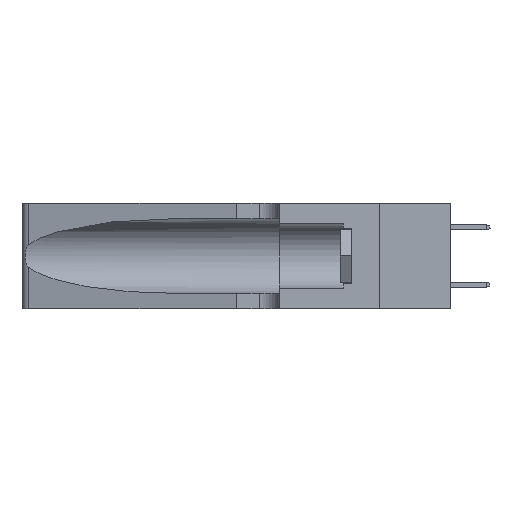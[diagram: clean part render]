
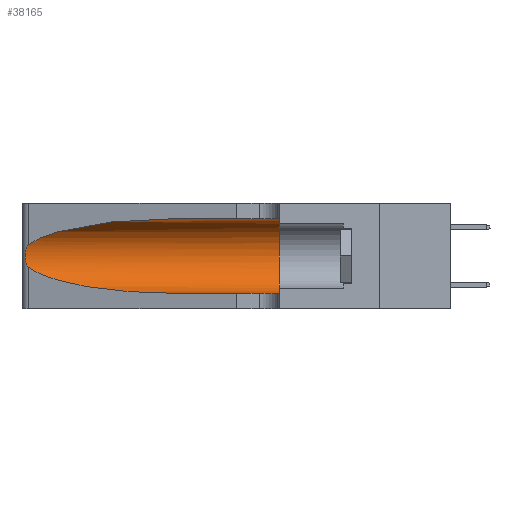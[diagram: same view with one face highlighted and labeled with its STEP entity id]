
A CAD part, left-side view. The second image highlights one B-rep face of the part: STEP entity #38165.
In plain terms, the highlighted cylindrical face has radius 3.308 mm (diameter 6.617 mm), a partial arc.
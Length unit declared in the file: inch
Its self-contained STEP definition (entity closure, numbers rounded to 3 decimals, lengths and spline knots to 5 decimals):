
#674 = CARTESIAN_POINT ( 'NONE',  ( 0.25487, 1.22718, 0.22369 ) ) ;
#1548 = CARTESIAN_POINT ( 'NONE',  ( 0.1305, 0.35, 0.31525 ) ) ;
#2005 = CARTESIAN_POINT ( 'NONE',  ( 0.1305, 1.61858, 0.05475 ) ) ;
#2157 = CARTESIAN_POINT ( 'NONE',  ( 0.2373, 1.15595, 0.08982 ) ) ;
#2640 = CARTESIAN_POINT ( 'NONE',  ( 0.18966, 0.96281, 0.31525 ) ) ;
#2766 = ORIENTED_EDGE ( 'NONE', *, *, #16112, .T. ) ;
#3418 = ORIENTED_EDGE ( 'NONE', *, *, #40777, .T. ) ;
#3511 = CARTESIAN_POINT ( 'NONE',  ( 0.26017, 1.23833, 0.17102 ) ) ;
#4199 = VERTEX_POINT ( 'NONE', #1548 ) ;
#4525 = AXIS2_PLACEMENT_3D ( 'NONE', #36823, #33344, #7733 ) ;
#6346 = CARTESIAN_POINT ( 'NONE',  ( 0.2373, 1.15595, 0.28018 ) ) ;
#6961 = CARTESIAN_POINT ( 'NONE',  ( 0.26018, 1.23835, 0.19895 ) ) ;
#7003 = VERTEX_POINT ( 'NONE', #29132 ) ;
#7064 = VERTEX_POINT ( 'NONE', #30273 ) ;
#7733 = DIRECTION ( 'NONE',  ( 0., 0., 1. ) ) ;
#8592 = EDGE_CURVE ( 'NONE', #4199, #7003, #25182, .T. ) ;
#10224 = CARTESIAN_POINT ( 'NONE',  ( 0.25789, 1.23486, 0.15765 ) ) ;
#10460 = CARTESIAN_POINT ( 'NONE',  ( 0.25555, 1.22994, 0.2215 ) ) ;
#12903 = DIRECTION ( 'NONE',  ( 0., -1., 0. ) ) ;
#13152 = DIRECTION ( 'NONE',  ( 0., 0., -1. ) ) ;
#15577 =( BOUNDED_CURVE ( )  B_SPLINE_CURVE ( 3, ( #26675, #2157, #44427, #23227 ),
 .UNSPECIFIED., .F., .F. ) 
 B_SPLINE_CURVE_WITH_KNOTS ( ( 4, 4 ),
 ( 3.44316, 4.71239 ),
 .UNSPECIFIED. ) 
 CURVE ( )  GEOMETRIC_REPRESENTATION_ITEM ( )  RATIONAL_B_SPLINE_CURVE ( ( 1., 0.87, 0.87, 1. ) ) 
 REPRESENTATION_ITEM ( '' )  );
#15943 = CARTESIAN_POINT ( 'NONE',  ( 0.1305, 1.61858, 0.185 ) ) ;
#16112 = EDGE_CURVE ( 'NONE', #7064, #22006, #23537, .T. ) ;
#16828 = VECTOR ( 'NONE', #44669, 39.37008 ) ;
#17177 = CARTESIAN_POINT ( 'NONE',  ( 0.25787, 1.23484, 0.2124 ) ) ;
#19593 = CARTESIAN_POINT ( 'NONE',  ( 0.25487, 1.22718, 0.14631 ) ) ;
#20076 = B_SPLINE_CURVE_WITH_KNOTS ( 'NONE', 3,
 ( #23890, #10460, #20635, #17177, #45322, #6961, #20409, #27554, #3511, #31676, #10224, #24324, #21318, #38618 ),
 .UNSPECIFIED., .F., .F.,
 ( 4, 2, 2, 2, 2, 2, 4 ),
 ( 0., 0.00027, 0.00053, 0.00107, 0.0016, 0.00187, 0.00214 ),
 .UNSPECIFIED. ) ;
#20228 = CARTESIAN_POINT ( 'NONE',  ( 0.25487, 1.22718, 0.22369 ) ) ;
#20409 = CARTESIAN_POINT ( 'NONE',  ( 0.26075, 1.23896, 0.19203 ) ) ;
#20635 = CARTESIAN_POINT ( 'NONE',  ( 0.25639, 1.23184, 0.21858 ) ) ;
#21318 = CARTESIAN_POINT ( 'NONE',  ( 0.25555, 1.22993, 0.14849 ) ) ;
#22006 = VERTEX_POINT ( 'NONE', #674 ) ;
#23227 = CARTESIAN_POINT ( 'NONE',  ( 0.1305, 0.72297, 0.05475 ) ) ;
#23537 =( BOUNDED_CURVE ( )  B_SPLINE_CURVE ( 3, ( #27380, #2640, #6346, #20228 ),
 .UNSPECIFIED., .F., .F. ) 
 B_SPLINE_CURVE_WITH_KNOTS ( ( 4, 4 ),
 ( 1.5708, 2.84003 ),
 .UNSPECIFIED. ) 
 CURVE ( )  GEOMETRIC_REPRESENTATION_ITEM ( )  RATIONAL_B_SPLINE_CURVE ( ( 1., 0.87, 0.87, 1. ) ) 
 REPRESENTATION_ITEM ( '' )  );
#23542 = DIRECTION ( 'NONE',  ( 0., -1., 0. ) ) ;
#23890 = CARTESIAN_POINT ( 'NONE',  ( 0.25487, 1.22718, 0.22369 ) ) ;
#24324 = CARTESIAN_POINT ( 'NONE',  ( 0.25639, 1.23186, 0.15144 ) ) ;
#24605 = EDGE_LOOP ( 'NONE', ( #2766, #3418, #42504, #27431, #30433, #39760 ) ) ;
#24941 = VERTEX_POINT ( 'NONE', #27247 ) ;
#25182 = CIRCLE ( 'NONE', #4525, 0.13025 ) ;
#26675 = CARTESIAN_POINT ( 'NONE',  ( 0.25487, 1.22718, 0.14631 ) ) ;
#26790 = VECTOR ( 'NONE', #12903, 39.37008 ) ;
#27247 = CARTESIAN_POINT ( 'NONE',  ( 0.1305, 0.72297, 0.05475 ) ) ;
#27380 = CARTESIAN_POINT ( 'NONE',  ( 0.1305, 0.72297, 0.31525 ) ) ;
#27431 = ORIENTED_EDGE ( 'NONE', *, *, #28188, .T. ) ;
#27554 = CARTESIAN_POINT ( 'NONE',  ( 0.26075, 1.23896, 0.178 ) ) ;
#27809 = CARTESIAN_POINT ( 'NONE',  ( 0.1305, 1.61858, 0.31525 ) ) ;
#28188 = EDGE_CURVE ( 'NONE', #24941, #7003, #40365, .T. ) ;
#28290 = VERTEX_POINT ( 'NONE', #19593 ) ;
#29132 = CARTESIAN_POINT ( 'NONE',  ( 0.1305, 0.35, 0.05475 ) ) ;
#30113 = AXIS2_PLACEMENT_3D ( 'NONE', #15943, #23542, #13152 ) ;
#30205 = FACE_OUTER_BOUND ( 'NONE', #24605, .T. ) ;
#30273 = CARTESIAN_POINT ( 'NONE',  ( 0.1305, 0.72297, 0.31525 ) ) ;
#30433 = ORIENTED_EDGE ( 'NONE', *, *, #8592, .F. ) ;
#30435 = CYLINDRICAL_SURFACE ( 'NONE', #30113, 0.13025 ) ;
#31676 = CARTESIAN_POINT ( 'NONE',  ( 0.25856, 1.23593, 0.16098 ) ) ;
#33344 = DIRECTION ( 'NONE',  ( 0., 1., 0. ) ) ;
#35584 = EDGE_CURVE ( 'NONE', #7064, #4199, #45354, .T. ) ;
#36823 = CARTESIAN_POINT ( 'NONE',  ( 0.1305, 0.35, 0.185 ) ) ;
#38165 = ADVANCED_FACE ( 'NONE', ( #30205 ), #30435, .F. ) ;
#38618 = CARTESIAN_POINT ( 'NONE',  ( 0.25487, 1.22718, 0.14631 ) ) ;
#39760 = ORIENTED_EDGE ( 'NONE', *, *, #35584, .F. ) ;
#40365 = LINE ( 'NONE', #2005, #26790 ) ;
#40777 = EDGE_CURVE ( 'NONE', #22006, #28290, #20076, .T. ) ;
#42504 = ORIENTED_EDGE ( 'NONE', *, *, #44600, .T. ) ;
#44427 = CARTESIAN_POINT ( 'NONE',  ( 0.18966, 0.96281, 0.05475 ) ) ;
#44600 = EDGE_CURVE ( 'NONE', #28290, #24941, #15577, .T. ) ;
#44669 = DIRECTION ( 'NONE',  ( 0., -1., 0. ) ) ;
#45322 = CARTESIAN_POINT ( 'NONE',  ( 0.25854, 1.2359, 0.20912 ) ) ;
#45354 = LINE ( 'NONE', #27809, #16828 ) ;
